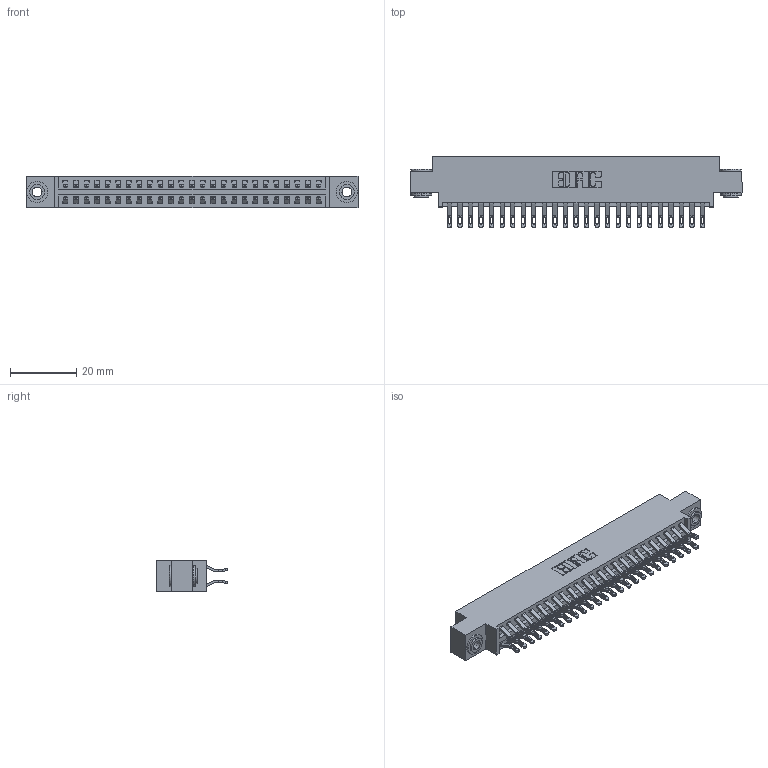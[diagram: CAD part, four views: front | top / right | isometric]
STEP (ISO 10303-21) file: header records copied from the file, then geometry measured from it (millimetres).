
FILE_DESCRIPTION (( 'STEP AP203' ), '1' );
FILE_NAME ('346-050-555-803.STEP', '2022-05-20T23:39:07', ( '' ), ( '' ), 'SwSTEP 2.0', 'SolidWorks 2020', '' );
FILE_SCHEMA (( 'CONFIG_CONTROL_DESIGN' ));
Length unit declared in the file: inch
Products named in the file (4): 346 Part_0.170 Offset - 0.156 Dia-TH; 346-050-555-803; 345-250-002_345-250-002-102; 345-292-001_555 Tail
Assembly tree (53 placements, depth 2):
  346-050-555-803
    346 Part_0.170 Offset - 0.156 Dia-TH
    345-292-001_555 Tail  x50
    345-250-002_345-250-002-102  x2
Bounding box: 99.95 x 21.46 x 9.4 mm (x, y, z)
Volume: 9605.9 mm3; surface area: 13882.1 mm2
Topology: 53 solids, 53 shells, 3078 faces, 9603 edges, 6398 vertices
Faces by surface type: plane 1754, cylinder 1316, cone 8
Entity records: 20128 total; most frequent: CARTESIAN_POINT 3359, ORIENTED_EDGE 3254, DIRECTION 3009, EDGE_CURVE 1627, LINE 1351, VECTOR 1351, VERTEX_POINT 1082, AXIS2_PLACEMENT_3D 829
